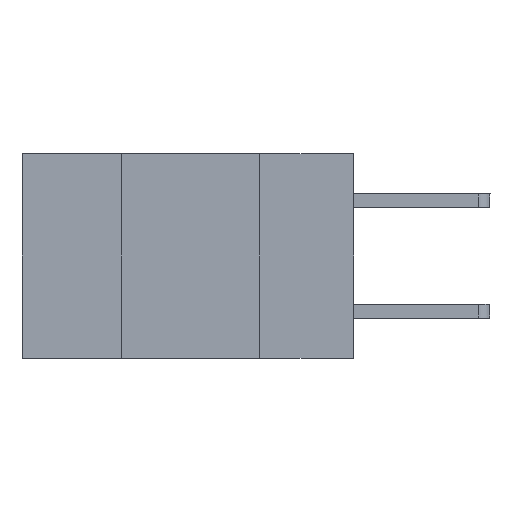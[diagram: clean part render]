
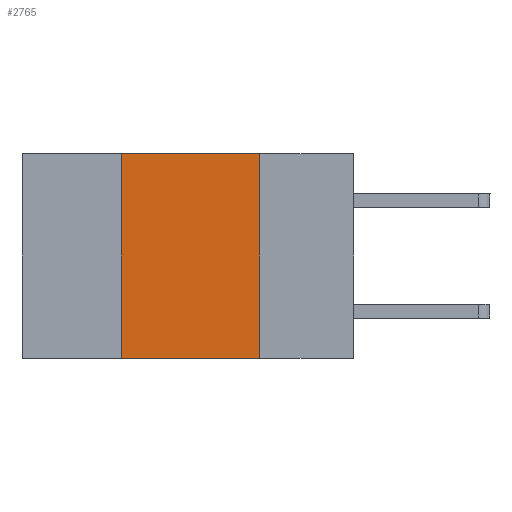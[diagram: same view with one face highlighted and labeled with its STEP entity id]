
A CAD part, left-side view. The second image highlights one B-rep face of the part: STEP entity #2765.
In plain terms, the highlighted planar face has unit normal (-1, 0, 0).
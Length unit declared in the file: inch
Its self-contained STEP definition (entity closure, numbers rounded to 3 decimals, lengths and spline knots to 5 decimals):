
#64 = ORIENTED_EDGE ( 'NONE', *, *, #5288, .F. ) ;
#726 = FACE_OUTER_BOUND ( 'NONE', #9858, .T. ) ;
#996 = DIRECTION ( 'NONE',  ( 0., -1., 0. ) ) ;
#1144 = EDGE_CURVE ( 'NONE', #6298, #8771, #1752, .T. ) ;
#1269 = LINE ( 'NONE', #6305, #8947 ) ;
#1286 = VECTOR ( 'NONE', #1372, 39.37008 ) ;
#1372 = DIRECTION ( 'NONE',  ( 0., 0., 1. ) ) ;
#1388 = EDGE_CURVE ( 'NONE', #3739, #2306, #9531, .T. ) ;
#1583 = DIRECTION ( 'NONE',  ( 1., 0., 0. ) ) ;
#1752 = LINE ( 'NONE', #4034, #7187 ) ;
#2094 = LINE ( 'NONE', #4487, #6975 ) ;
#2306 = VERTEX_POINT ( 'NONE', #5723 ) ;
#2765 = ADVANCED_FACE ( 'NONE', ( #726 ), #6514, .F. ) ;
#3372 = DIRECTION ( 'NONE',  ( 0., 0., -1. ) ) ;
#3739 = VERTEX_POINT ( 'NONE', #8308 ) ;
#3764 = DIRECTION ( 'NONE',  ( 0., -1., 0. ) ) ;
#4034 = CARTESIAN_POINT ( 'NONE',  ( 0., 0.17, 0. ) ) ;
#4487 = CARTESIAN_POINT ( 'NONE',  ( 0., 0.6, 0. ) ) ;
#5253 = ORIENTED_EDGE ( 'NONE', *, *, #1144, .F. ) ;
#5288 = EDGE_CURVE ( 'NONE', #2306, #6298, #2094, .T. ) ;
#5595 = CARTESIAN_POINT ( 'NONE',  ( 0., 0.42, 0. ) ) ;
#5723 = CARTESIAN_POINT ( 'NONE',  ( 0., 0.42, 0. ) ) ;
#6298 = VERTEX_POINT ( 'NONE', #8138 ) ;
#6305 = CARTESIAN_POINT ( 'NONE',  ( 0., 0.6, -0.37 ) ) ;
#6485 = AXIS2_PLACEMENT_3D ( 'NONE', #6607, #1583, #3372 ) ;
#6514 = PLANE ( 'NONE',  #6485 ) ;
#6607 = CARTESIAN_POINT ( 'NONE',  ( 0., 0.6, 0. ) ) ;
#6975 = VECTOR ( 'NONE', #996, 39.37008 ) ;
#7091 = ORIENTED_EDGE ( 'NONE', *, *, #9530, .T. ) ;
#7187 = VECTOR ( 'NONE', #7492, 39.37008 ) ;
#7492 = DIRECTION ( 'NONE',  ( 0., 0., -1. ) ) ;
#8138 = CARTESIAN_POINT ( 'NONE',  ( 0., 0.17, 0. ) ) ;
#8308 = CARTESIAN_POINT ( 'NONE',  ( 0., 0.42, -0.37 ) ) ;
#8771 = VERTEX_POINT ( 'NONE', #9485 ) ;
#8947 = VECTOR ( 'NONE', #3764, 39.37008 ) ;
#9485 = CARTESIAN_POINT ( 'NONE',  ( 0., 0.17, -0.37 ) ) ;
#9530 = EDGE_CURVE ( 'NONE', #3739, #8771, #1269, .T. ) ;
#9531 = LINE ( 'NONE', #5595, #1286 ) ;
#9858 = EDGE_LOOP ( 'NONE', ( #5253, #64, #10229, #7091 ) ) ;
#10229 = ORIENTED_EDGE ( 'NONE', *, *, #1388, .F. ) ;
